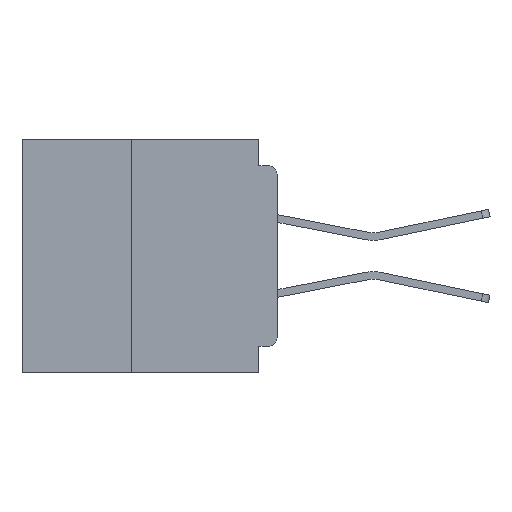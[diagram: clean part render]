
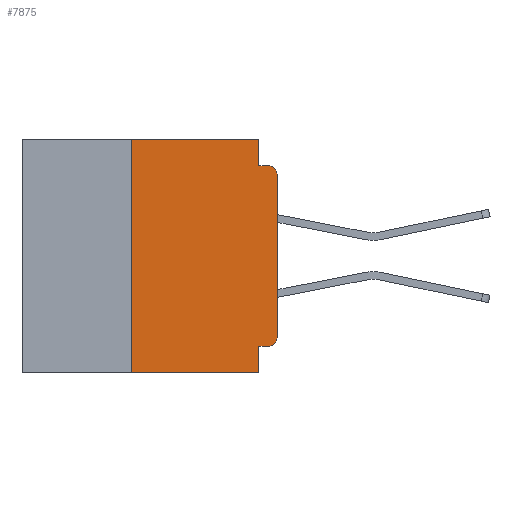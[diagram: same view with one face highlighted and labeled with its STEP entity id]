
A CAD part, left-side view. The second image highlights one B-rep face of the part: STEP entity #7875.
In plain terms, the highlighted planar face has unit normal (-1, 0, 0).
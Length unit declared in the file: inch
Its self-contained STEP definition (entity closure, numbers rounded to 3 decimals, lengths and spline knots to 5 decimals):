
#993 = VECTOR ( 'NONE', #21058, 39.37008 ) ;
#1142 = ORIENTED_EDGE ( 'NONE', *, *, #30203, .T. ) ;
#2169 = DIRECTION ( 'NONE',  ( 0., 0., -1. ) ) ;
#2449 = VERTEX_POINT ( 'NONE', #3595 ) ;
#2802 = VECTOR ( 'NONE', #39129, 39.37008 ) ;
#3595 = CARTESIAN_POINT ( 'NONE',  ( 0., 0.031, -0.045 ) ) ;
#4178 = EDGE_CURVE ( 'NONE', #14212, #26423, #23336, .T. ) ;
#4495 = ORIENTED_EDGE ( 'NONE', *, *, #4725, .F. ) ;
#4725 = EDGE_CURVE ( 'NONE', #17335, #34676, #11553, .T. ) ;
#5682 = AXIS2_PLACEMENT_3D ( 'NONE', #9749, #32610, #13072 ) ;
#6248 = VECTOR ( 'NONE', #19757, 39.37008 ) ;
#6441 = ORIENTED_EDGE ( 'NONE', *, *, #37205, .F. ) ;
#6924 = CARTESIAN_POINT ( 'NONE',  ( 0., 0.015, -0.355 ) ) ;
#7294 = CARTESIAN_POINT ( 'NONE',  ( 0., 0., -0.355 ) ) ;
#7504 = VERTEX_POINT ( 'NONE', #29699 ) ;
#7875 = ADVANCED_FACE ( 'NONE', ( #18937 ), #37927, .F. ) ;
#9205 = CARTESIAN_POINT ( 'NONE',  ( 0., 0.031, 0. ) ) ;
#9749 = CARTESIAN_POINT ( 'NONE',  ( 0., 0.015, -0.06 ) ) ;
#11553 = LINE ( 'NONE', #13051, #2802 ) ;
#12405 = VERTEX_POINT ( 'NONE', #14580 ) ;
#13051 = CARTESIAN_POINT ( 'NONE',  ( 0., 0.25, -0.4 ) ) ;
#13072 = DIRECTION ( 'NONE',  ( 0., 0., -1. ) ) ;
#13496 = ORIENTED_EDGE ( 'NONE', *, *, #14736, .T. ) ;
#13513 = DIRECTION ( 'NONE',  ( -1., 0., 0. ) ) ;
#13758 = LINE ( 'NONE', #7294, #21426 ) ;
#14164 = ORIENTED_EDGE ( 'NONE', *, *, #18492, .F. ) ;
#14212 = VERTEX_POINT ( 'NONE', #6924 ) ;
#14580 = CARTESIAN_POINT ( 'NONE',  ( 0., 0.031, -0.4 ) ) ;
#14736 = EDGE_CURVE ( 'NONE', #35393, #16150, #38251, .T. ) ;
#14935 = EDGE_CURVE ( 'NONE', #14212, #7504, #13758, .T. ) ;
#15268 = DIRECTION ( 'NONE',  ( 0., -1., 0. ) ) ;
#16150 = VERTEX_POINT ( 'NONE', #20769 ) ;
#16175 = LINE ( 'NONE', #9205, #41183 ) ;
#16500 = EDGE_CURVE ( 'NONE', #26423, #35393, #23650, .T. ) ;
#17335 = VERTEX_POINT ( 'NONE', #30671 ) ;
#17763 = CARTESIAN_POINT ( 'NONE',  ( 0., 0.437, 0. ) ) ;
#18492 = EDGE_CURVE ( 'NONE', #7504, #12405, #31652, .T. ) ;
#18937 = FACE_OUTER_BOUND ( 'NONE', #21364, .T. ) ;
#19518 = CARTESIAN_POINT ( 'NONE',  ( 0., 0.031, -0.4 ) ) ;
#19757 = DIRECTION ( 'NONE',  ( 0., 0., 1. ) ) ;
#20302 = EDGE_CURVE ( 'NONE', #29716, #2449, #16175, .T. ) ;
#20769 = CARTESIAN_POINT ( 'NONE',  ( 0., 0.015, -0.045 ) ) ;
#21058 = DIRECTION ( 'NONE',  ( 0., -1., 0. ) ) ;
#21364 = EDGE_LOOP ( 'NONE', ( #41310, #13496, #6441, #40085, #33746, #4495, #1142, #14164, #42122, #38072 ) ) ;
#21426 = VECTOR ( 'NONE', #39982, 39.37008 ) ;
#21635 = AXIS2_PLACEMENT_3D ( 'NONE', #33058, #13513, #36301 ) ;
#21843 = DIRECTION ( 'NONE',  ( 1., 0., 0. ) ) ;
#22935 = VECTOR ( 'NONE', #15268, 39.37008 ) ;
#23336 = CIRCLE ( 'NONE', #21635, 0.015 ) ;
#23650 = LINE ( 'NONE', #35989, #6248 ) ;
#23800 = VECTOR ( 'NONE', #36241, 39.37008 ) ;
#23983 = VECTOR ( 'NONE', #42311, 39.37008 ) ;
#25684 = EDGE_CURVE ( 'NONE', #34676, #29716, #27192, .T. ) ;
#26423 = VERTEX_POINT ( 'NONE', #34972 ) ;
#27192 = LINE ( 'NONE', #17763, #993 ) ;
#29699 = CARTESIAN_POINT ( 'NONE',  ( 0., 0.031, -0.355 ) ) ;
#29716 = VERTEX_POINT ( 'NONE', #40592 ) ;
#30203 = EDGE_CURVE ( 'NONE', #17335, #12405, #31612, .T. ) ;
#30671 = CARTESIAN_POINT ( 'NONE',  ( 0., 0.25, -0.4 ) ) ;
#31534 = CARTESIAN_POINT ( 'NONE',  ( 0., 0.437, 0. ) ) ;
#31612 = LINE ( 'NONE', #34802, #22935 ) ;
#31652 = LINE ( 'NONE', #19518, #23983 ) ;
#32055 = DIRECTION ( 'NONE',  ( 0., 0., -1. ) ) ;
#32485 = LINE ( 'NONE', #36108, #23800 ) ;
#32610 = DIRECTION ( 'NONE',  ( -1., 0., 0. ) ) ;
#33058 = CARTESIAN_POINT ( 'NONE',  ( 0., 0.015, -0.34 ) ) ;
#33193 = AXIS2_PLACEMENT_3D ( 'NONE', #31534, #21843, #2169 ) ;
#33746 = ORIENTED_EDGE ( 'NONE', *, *, #25684, .F. ) ;
#34228 = CARTESIAN_POINT ( 'NONE',  ( 0., 0.25, 0. ) ) ;
#34676 = VERTEX_POINT ( 'NONE', #34228 ) ;
#34802 = CARTESIAN_POINT ( 'NONE',  ( 0., 0.437, -0.4 ) ) ;
#34972 = CARTESIAN_POINT ( 'NONE',  ( 0., 0., -0.34 ) ) ;
#35393 = VERTEX_POINT ( 'NONE', #37713 ) ;
#35989 = CARTESIAN_POINT ( 'NONE',  ( 0., 0., 0. ) ) ;
#36108 = CARTESIAN_POINT ( 'NONE',  ( 0., 0., -0.045 ) ) ;
#36241 = DIRECTION ( 'NONE',  ( 0., -1., 0. ) ) ;
#36301 = DIRECTION ( 'NONE',  ( 0., 0., -1. ) ) ;
#37205 = EDGE_CURVE ( 'NONE', #2449, #16150, #32485, .T. ) ;
#37713 = CARTESIAN_POINT ( 'NONE',  ( 0., 0., -0.06 ) ) ;
#37927 = PLANE ( 'NONE',  #33193 ) ;
#38072 = ORIENTED_EDGE ( 'NONE', *, *, #4178, .T. ) ;
#38251 = CIRCLE ( 'NONE', #5682, 0.015 ) ;
#39129 = DIRECTION ( 'NONE',  ( 0., 0., 1. ) ) ;
#39982 = DIRECTION ( 'NONE',  ( 0., 1., 0. ) ) ;
#40085 = ORIENTED_EDGE ( 'NONE', *, *, #20302, .F. ) ;
#40592 = CARTESIAN_POINT ( 'NONE',  ( 0., 0.031, 0. ) ) ;
#41183 = VECTOR ( 'NONE', #32055, 39.37008 ) ;
#41310 = ORIENTED_EDGE ( 'NONE', *, *, #16500, .T. ) ;
#42122 = ORIENTED_EDGE ( 'NONE', *, *, #14935, .F. ) ;
#42311 = DIRECTION ( 'NONE',  ( 0., 0., -1. ) ) ;
